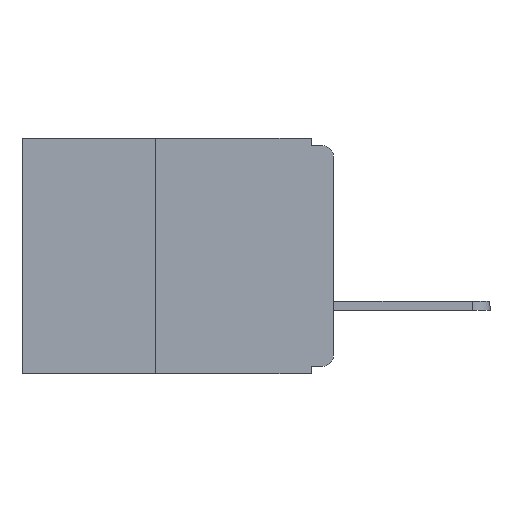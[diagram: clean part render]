
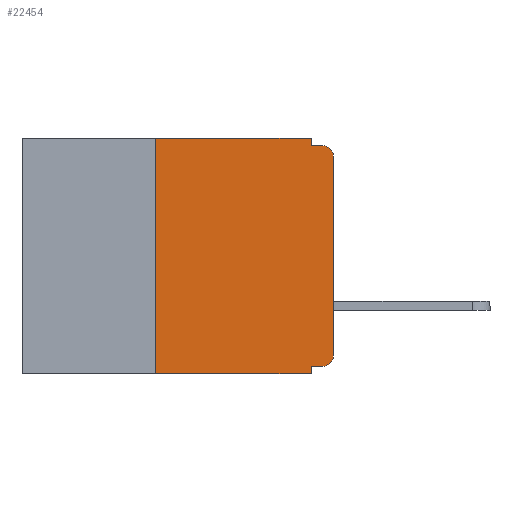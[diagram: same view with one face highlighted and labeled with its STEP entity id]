
A CAD part, left-side view. The second image highlights one B-rep face of the part: STEP entity #22454.
In plain terms, the highlighted planar face has unit normal (-1, 0, 0).
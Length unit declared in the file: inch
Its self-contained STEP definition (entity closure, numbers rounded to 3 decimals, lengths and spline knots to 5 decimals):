
#1137 = CARTESIAN_POINT ( 'NONE',  ( 0., 0.437, 0. ) ) ;
#1211 = CARTESIAN_POINT ( 'NONE',  ( 0., 0.031, -0.33 ) ) ;
#1323 = CARTESIAN_POINT ( 'NONE',  ( 0., 0.031, -0.01 ) ) ;
#1665 = DIRECTION ( 'NONE',  ( 0., 0., -1. ) ) ;
#1729 = CARTESIAN_POINT ( 'NONE',  ( 0., 0.031, 0. ) ) ;
#2043 = VERTEX_POINT ( 'NONE', #1323 ) ;
#2443 = PLANE ( 'NONE',  #14740 ) ;
#2471 = VECTOR ( 'NONE', #10217, 39.37008 ) ;
#2880 = VECTOR ( 'NONE', #1665, 39.37008 ) ;
#3124 = DIRECTION ( 'NONE',  ( 0., 0., -1. ) ) ;
#3339 = VERTEX_POINT ( 'NONE', #7000 ) ;
#3391 = LINE ( 'NONE', #17250, #17410 ) ;
#3666 = EDGE_LOOP ( 'NONE', ( #11574, #12153, #14428, #22629, #20640, #16385, #15010, #20366, #3827, #9313 ) ) ;
#3761 = EDGE_CURVE ( 'NONE', #11687, #3339, #3391, .T. ) ;
#3827 = ORIENTED_EDGE ( 'NONE', *, *, #4456, .F. ) ;
#4077 = VERTEX_POINT ( 'NONE', #21215 ) ;
#4243 = CARTESIAN_POINT ( 'NONE',  ( 0., 0.015, -0.305 ) ) ;
#4365 = CARTESIAN_POINT ( 'NONE',  ( 0., 0.437, 0. ) ) ;
#4456 = EDGE_CURVE ( 'NONE', #18728, #5000, #12873, .T. ) ;
#4683 = CARTESIAN_POINT ( 'NONE',  ( 0., 0., -0.01 ) ) ;
#4698 = CARTESIAN_POINT ( 'NONE',  ( 0., 0., 0. ) ) ;
#5000 = VERTEX_POINT ( 'NONE', #16419 ) ;
#5093 = LINE ( 'NONE', #1211, #18484 ) ;
#5152 = FACE_OUTER_BOUND ( 'NONE', #3666, .T. ) ;
#6100 = DIRECTION ( 'NONE',  ( 0., 0., -1. ) ) ;
#6204 = DIRECTION ( 'NONE',  ( 0., 0., -1. ) ) ;
#6356 = EDGE_CURVE ( 'NONE', #14783, #23769, #10172, .T. ) ;
#6456 = VERTEX_POINT ( 'NONE', #14845 ) ;
#7000 = CARTESIAN_POINT ( 'NONE',  ( 0., 0.25, 0. ) ) ;
#7318 = EDGE_CURVE ( 'NONE', #6456, #2043, #12706, .T. ) ;
#7874 = CIRCLE ( 'NONE', #15043, 0.015 ) ;
#8040 = LINE ( 'NONE', #9470, #17724 ) ;
#8527 = EDGE_CURVE ( 'NONE', #14631, #14783, #17411, .T. ) ;
#9313 = ORIENTED_EDGE ( 'NONE', *, *, #22997, .T. ) ;
#9470 = CARTESIAN_POINT ( 'NONE',  ( 0., 0.437, -0.33 ) ) ;
#9816 = CARTESIAN_POINT ( 'NONE',  ( 0., 0., -0.305 ) ) ;
#10062 = CARTESIAN_POINT ( 'NONE',  ( 0., 0., -0.32 ) ) ;
#10172 = CIRCLE ( 'NONE', #23562, 0.015 ) ;
#10217 = DIRECTION ( 'NONE',  ( 0., 1., 0. ) ) ;
#11438 = VECTOR ( 'NONE', #15619, 39.37008 ) ;
#11511 = CARTESIAN_POINT ( 'NONE',  ( 0., 0.25, -0.33 ) ) ;
#11574 = ORIENTED_EDGE ( 'NONE', *, *, #8527, .T. ) ;
#11687 = VERTEX_POINT ( 'NONE', #11511 ) ;
#12096 = CARTESIAN_POINT ( 'NONE',  ( 0., 0.015, -0.01 ) ) ;
#12153 = ORIENTED_EDGE ( 'NONE', *, *, #6356, .T. ) ;
#12244 = DIRECTION ( 'NONE',  ( 0., -1., 0. ) ) ;
#12628 = VECTOR ( 'NONE', #15633, 39.37008 ) ;
#12706 = LINE ( 'NONE', #1729, #2880 ) ;
#12873 = LINE ( 'NONE', #10062, #2471 ) ;
#13550 = LINE ( 'NONE', #1137, #22579 ) ;
#13742 = LINE ( 'NONE', #4683, #11438 ) ;
#14306 = DIRECTION ( 'NONE',  ( 0., 0., 1. ) ) ;
#14428 = ORIENTED_EDGE ( 'NONE', *, *, #14782, .F. ) ;
#14631 = VERTEX_POINT ( 'NONE', #9816 ) ;
#14740 = AXIS2_PLACEMENT_3D ( 'NONE', #4365, #17096, #6204 ) ;
#14782 = EDGE_CURVE ( 'NONE', #2043, #23769, #13742, .T. ) ;
#14783 = VERTEX_POINT ( 'NONE', #21065 ) ;
#14845 = CARTESIAN_POINT ( 'NONE',  ( 0., 0.031, 0. ) ) ;
#15010 = ORIENTED_EDGE ( 'NONE', *, *, #21222, .T. ) ;
#15043 = AXIS2_PLACEMENT_3D ( 'NONE', #4243, #17003, #6100 ) ;
#15619 = DIRECTION ( 'NONE',  ( 0., -1., 0. ) ) ;
#15633 = DIRECTION ( 'NONE',  ( 0., 0., 1. ) ) ;
#16086 = EDGE_CURVE ( 'NONE', #5000, #4077, #5093, .T. ) ;
#16385 = ORIENTED_EDGE ( 'NONE', *, *, #3761, .F. ) ;
#16419 = CARTESIAN_POINT ( 'NONE',  ( 0., 0.031, -0.32 ) ) ;
#16804 = DIRECTION ( 'NONE',  ( 0., 0., -1. ) ) ;
#16859 = DIRECTION ( 'NONE',  ( -1., 0., 0. ) ) ;
#16886 = CARTESIAN_POINT ( 'NONE',  ( 0., 0.015, -0.025 ) ) ;
#17003 = DIRECTION ( 'NONE',  ( -1., 0., 0. ) ) ;
#17096 = DIRECTION ( 'NONE',  ( 1., 0., 0. ) ) ;
#17250 = CARTESIAN_POINT ( 'NONE',  ( 0., 0.25, -0.33 ) ) ;
#17410 = VECTOR ( 'NONE', #14306, 39.37008 ) ;
#17411 = LINE ( 'NONE', #4698, #12628 ) ;
#17724 = VECTOR ( 'NONE', #20320, 39.37008 ) ;
#18484 = VECTOR ( 'NONE', #3124, 39.37008 ) ;
#18728 = VERTEX_POINT ( 'NONE', #22465 ) ;
#20320 = DIRECTION ( 'NONE',  ( 0., -1., 0. ) ) ;
#20358 = EDGE_CURVE ( 'NONE', #3339, #6456, #13550, .T. ) ;
#20366 = ORIENTED_EDGE ( 'NONE', *, *, #16086, .F. ) ;
#20640 = ORIENTED_EDGE ( 'NONE', *, *, #20358, .F. ) ;
#21065 = CARTESIAN_POINT ( 'NONE',  ( 0., 0., -0.025 ) ) ;
#21215 = CARTESIAN_POINT ( 'NONE',  ( 0., 0.031, -0.33 ) ) ;
#21222 = EDGE_CURVE ( 'NONE', #11687, #4077, #8040, .T. ) ;
#22454 = ADVANCED_FACE ( 'NONE', ( #5152 ), #2443, .F. ) ;
#22465 = CARTESIAN_POINT ( 'NONE',  ( 0., 0.015, -0.32 ) ) ;
#22579 = VECTOR ( 'NONE', #12244, 39.37008 ) ;
#22629 = ORIENTED_EDGE ( 'NONE', *, *, #7318, .F. ) ;
#22997 = EDGE_CURVE ( 'NONE', #18728, #14631, #7874, .T. ) ;
#23562 = AXIS2_PLACEMENT_3D ( 'NONE', #16886, #16859, #16804 ) ;
#23769 = VERTEX_POINT ( 'NONE', #12096 ) ;
